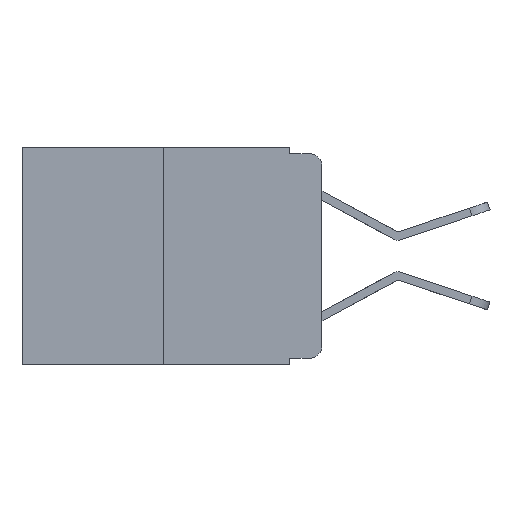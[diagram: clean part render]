
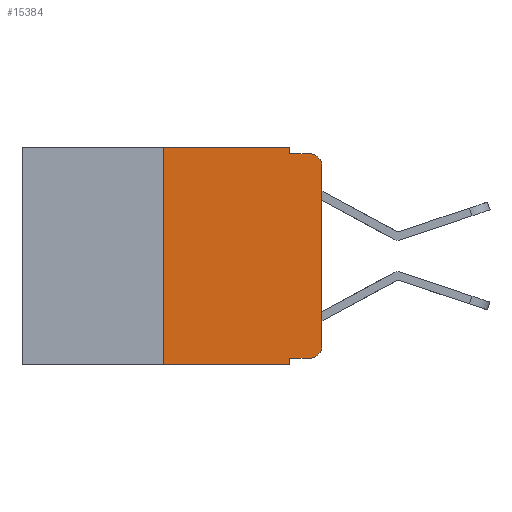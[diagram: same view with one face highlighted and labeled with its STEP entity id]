
A CAD part, left-side view. The second image highlights one B-rep face of the part: STEP entity #15384.
In plain terms, the highlighted planar face has unit normal (-1, 0, 0).
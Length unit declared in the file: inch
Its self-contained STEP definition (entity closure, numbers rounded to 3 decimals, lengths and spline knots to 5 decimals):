
#28 = DIRECTION ( 'NONE',  ( 0., 0., 1. ) ) ;
#163 = ORIENTED_EDGE ( 'NONE', *, *, #8329, .F. ) ;
#1654 = DIRECTION ( 'NONE',  ( 0., 0., -1. ) ) ;
#2156 = VECTOR ( 'NONE', #19724, 39.37008 ) ;
#2178 = EDGE_CURVE ( 'NONE', #9294, #18871, #8396, .T. ) ;
#2257 = DIRECTION ( 'NONE',  ( 0., -1., 0. ) ) ;
#2942 = VERTEX_POINT ( 'NONE', #19719 ) ;
#3136 = CARTESIAN_POINT ( 'NONE',  ( 0., 0.473, 0. ) ) ;
#3926 = CARTESIAN_POINT ( 'NONE',  ( 0., 0.473, 0. ) ) ;
#3982 = VERTEX_POINT ( 'NONE', #4740 ) ;
#4440 = ORIENTED_EDGE ( 'NONE', *, *, #15216, .T. ) ;
#4740 = CARTESIAN_POINT ( 'NONE',  ( 0., 0., -0.313 ) ) ;
#4784 = CARTESIAN_POINT ( 'NONE',  ( 0., 0.02, -0.313 ) ) ;
#4910 = ORIENTED_EDGE ( 'NONE', *, *, #2178, .T. ) ;
#4935 = DIRECTION ( 'NONE',  ( 1., 0., 0. ) ) ;
#4957 = VECTOR ( 'NONE', #28, 39.37008 ) ;
#5250 = VERTEX_POINT ( 'NONE', #20674 ) ;
#6145 = LINE ( 'NONE', #23892, #4957 ) ;
#6588 = AXIS2_PLACEMENT_3D ( 'NONE', #13020, #18892, #1654 ) ;
#7134 = DIRECTION ( 'NONE',  ( 0., -1., 0. ) ) ;
#7389 = ORIENTED_EDGE ( 'NONE', *, *, #17806, .T. ) ;
#7630 = DIRECTION ( 'NONE',  ( 0., -1., 0. ) ) ;
#8143 = VECTOR ( 'NONE', #7630, 39.37008 ) ;
#8329 = EDGE_CURVE ( 'NONE', #9966, #5250, #14944, .T. ) ;
#8396 = CIRCLE ( 'NONE', #6588, 0.02 ) ;
#8751 = LINE ( 'NONE', #18998, #8143 ) ;
#8784 = ORIENTED_EDGE ( 'NONE', *, *, #18451, .F. ) ;
#9014 = VERTEX_POINT ( 'NONE', #16893 ) ;
#9294 = VERTEX_POINT ( 'NONE', #16687 ) ;
#9376 = VERTEX_POINT ( 'NONE', #14910 ) ;
#9966 = VERTEX_POINT ( 'NONE', #12027 ) ;
#10321 = CIRCLE ( 'NONE', #23121, 0.02 ) ;
#10445 = CARTESIAN_POINT ( 'NONE',  ( 0., 0.051, -0.343 ) ) ;
#10783 = CARTESIAN_POINT ( 'NONE',  ( 0., 0.473, -0.343 ) ) ;
#10977 = DIRECTION ( 'NONE',  ( 0., 0., 1. ) ) ;
#11086 = EDGE_CURVE ( 'NONE', #9376, #17032, #6145, .T. ) ;
#11376 = VECTOR ( 'NONE', #16959, 39.37008 ) ;
#11572 = LINE ( 'NONE', #10783, #21680 ) ;
#11731 = ORIENTED_EDGE ( 'NONE', *, *, #11086, .F. ) ;
#12027 = CARTESIAN_POINT ( 'NONE',  ( 0., 0.051, 0. ) ) ;
#12188 = VECTOR ( 'NONE', #2257, 39.37008 ) ;
#12687 = DIRECTION ( 'NONE',  ( 0., -1., 0. ) ) ;
#13020 = CARTESIAN_POINT ( 'NONE',  ( 0., 0.02, -0.03 ) ) ;
#13097 = ORIENTED_EDGE ( 'NONE', *, *, #24229, .F. ) ;
#13331 = FACE_OUTER_BOUND ( 'NONE', #18759, .T. ) ;
#13471 = EDGE_CURVE ( 'NONE', #17032, #9966, #13699, .T. ) ;
#13699 = LINE ( 'NONE', #3926, #12188 ) ;
#13868 = EDGE_CURVE ( 'NONE', #9376, #18939, #11572, .T. ) ;
#14174 = DIRECTION ( 'NONE',  ( 0., 0., -1. ) ) ;
#14294 = CARTESIAN_POINT ( 'NONE',  ( 0., 0.02, -0.01 ) ) ;
#14910 = CARTESIAN_POINT ( 'NONE',  ( 0., 0.25, -0.343 ) ) ;
#14944 = LINE ( 'NONE', #21456, #2156 ) ;
#15216 = EDGE_CURVE ( 'NONE', #9014, #3982, #10321, .T. ) ;
#15384 = ADVANCED_FACE ( 'NONE', ( #13331 ), #16337, .F. ) ;
#15424 = EDGE_CURVE ( 'NONE', #3982, #9294, #21282, .T. ) ;
#15868 = AXIS2_PLACEMENT_3D ( 'NONE', #3136, #4935, #20130 ) ;
#16337 = PLANE ( 'NONE',  #15868 ) ;
#16687 = CARTESIAN_POINT ( 'NONE',  ( 0., 0., -0.03 ) ) ;
#16801 = CARTESIAN_POINT ( 'NONE',  ( 0., 0.051, 0. ) ) ;
#16893 = CARTESIAN_POINT ( 'NONE',  ( 0., 0.02, -0.333 ) ) ;
#16959 = DIRECTION ( 'NONE',  ( 0., 0., -1. ) ) ;
#17032 = VERTEX_POINT ( 'NONE', #19791 ) ;
#17272 = ORIENTED_EDGE ( 'NONE', *, *, #13471, .F. ) ;
#17806 = EDGE_CURVE ( 'NONE', #2942, #9014, #19397, .T. ) ;
#18451 = EDGE_CURVE ( 'NONE', #2942, #18939, #21802, .T. ) ;
#18556 = CARTESIAN_POINT ( 'NONE',  ( 0., 0., 0. ) ) ;
#18759 = EDGE_LOOP ( 'NONE', ( #23221, #4910, #13097, #163, #17272, #11731, #18948, #8784, #7389, #4440 ) ) ;
#18871 = VERTEX_POINT ( 'NONE', #14294 ) ;
#18892 = DIRECTION ( 'NONE',  ( -1., 0., 0. ) ) ;
#18939 = VERTEX_POINT ( 'NONE', #10445 ) ;
#18948 = ORIENTED_EDGE ( 'NONE', *, *, #13868, .T. ) ;
#18998 = CARTESIAN_POINT ( 'NONE',  ( 0., 0.051, -0.01 ) ) ;
#19397 = LINE ( 'NONE', #24199, #23244 ) ;
#19520 = VECTOR ( 'NONE', #10977, 39.37008 ) ;
#19719 = CARTESIAN_POINT ( 'NONE',  ( 0., 0.051, -0.333 ) ) ;
#19724 = DIRECTION ( 'NONE',  ( 0., 0., -1. ) ) ;
#19791 = CARTESIAN_POINT ( 'NONE',  ( 0., 0.25, 0. ) ) ;
#20130 = DIRECTION ( 'NONE',  ( 0., 0., -1. ) ) ;
#20674 = CARTESIAN_POINT ( 'NONE',  ( 0., 0.051, -0.01 ) ) ;
#21282 = LINE ( 'NONE', #18556, #19520 ) ;
#21456 = CARTESIAN_POINT ( 'NONE',  ( 0., 0.051, 0. ) ) ;
#21680 = VECTOR ( 'NONE', #7134, 39.37008 ) ;
#21802 = LINE ( 'NONE', #16801, #11376 ) ;
#23121 = AXIS2_PLACEMENT_3D ( 'NONE', #4784, #23690, #14174 ) ;
#23221 = ORIENTED_EDGE ( 'NONE', *, *, #15424, .T. ) ;
#23244 = VECTOR ( 'NONE', #12687, 39.37008 ) ;
#23690 = DIRECTION ( 'NONE',  ( -1., 0., 0. ) ) ;
#23892 = CARTESIAN_POINT ( 'NONE',  ( 0., 0.25, 0. ) ) ;
#24199 = CARTESIAN_POINT ( 'NONE',  ( 0., 0.051, -0.333 ) ) ;
#24229 = EDGE_CURVE ( 'NONE', #5250, #18871, #8751, .T. ) ;
